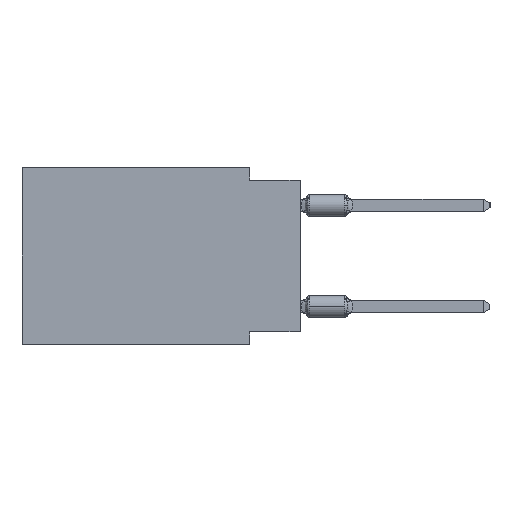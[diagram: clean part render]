
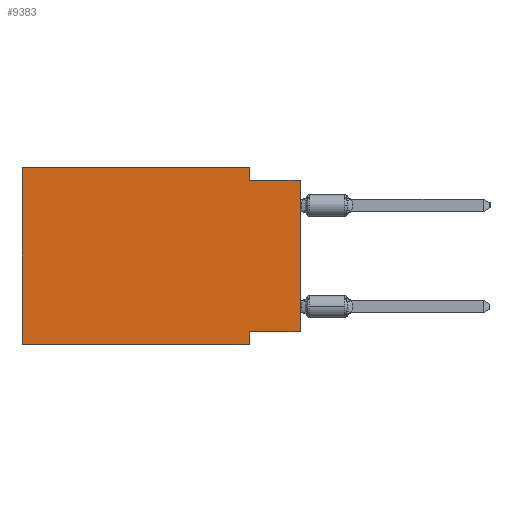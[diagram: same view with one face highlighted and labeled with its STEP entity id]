
A CAD part, left-side view. The second image highlights one B-rep face of the part: STEP entity #9383.
In plain terms, the highlighted planar face has unit normal (-1, 0, 0).
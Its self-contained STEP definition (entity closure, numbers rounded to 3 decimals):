
#22 = LINE ( 'NONE', #15636, #12544 ) ;
#81 = VERTEX_POINT ( 'NONE', #32226 ) ;
#788 = EDGE_LOOP ( 'NONE', ( #20646, #19501, #6830, #11508, #5586, #4826, #31515, #23797 ) ) ;
#2620 = EDGE_CURVE ( 'NONE', #30941, #81, #27450, .T. ) ;
#4728 = CARTESIAN_POINT ( 'NONE',  ( 0., 13.97, -8.89 ) ) ;
#4826 = ORIENTED_EDGE ( 'NONE', *, *, #15686, .T. ) ;
#4896 = CARTESIAN_POINT ( 'NONE',  ( 0., 0., -8.255 ) ) ;
#5426 = VECTOR ( 'NONE', #12375, 1000. ) ;
#5586 = ORIENTED_EDGE ( 'NONE', *, *, #15445, .F. ) ;
#5621 = LINE ( 'NONE', #7819, #14363 ) ;
#6531 = VECTOR ( 'NONE', #18871, 1000. ) ;
#6609 = LINE ( 'NONE', #20182, #5426 ) ;
#6830 = ORIENTED_EDGE ( 'NONE', *, *, #10685, .F. ) ;
#7659 = VECTOR ( 'NONE', #31366, 1000. ) ;
#7726 = LINE ( 'NONE', #18282, #7659 ) ;
#7819 = CARTESIAN_POINT ( 'NONE',  ( 0., 0., -0.635 ) ) ;
#7893 = VERTEX_POINT ( 'NONE', #19875 ) ;
#8503 = LINE ( 'NONE', #11541, #6531 ) ;
#9383 = ADVANCED_FACE ( 'NONE', ( #26511 ), #13760, .F. ) ;
#9607 = EDGE_CURVE ( 'NONE', #19633, #23455, #6609, .T. ) ;
#9655 = VERTEX_POINT ( 'NONE', #4896 ) ;
#10685 = EDGE_CURVE ( 'NONE', #23455, #26464, #8503, .T. ) ;
#10727 = CARTESIAN_POINT ( 'NONE',  ( 0., 13.97, 0. ) ) ;
#11388 = EDGE_CURVE ( 'NONE', #9655, #30941, #7726, .T. ) ;
#11508 = ORIENTED_EDGE ( 'NONE', *, *, #9607, .F. ) ;
#11541 = CARTESIAN_POINT ( 'NONE',  ( 0., 2.54, 0. ) ) ;
#11980 = CARTESIAN_POINT ( 'NONE',  ( 0., 2.54, -8.89 ) ) ;
#12375 = DIRECTION ( 'NONE',  ( 0., -1., 0. ) ) ;
#12544 = VECTOR ( 'NONE', #31264, 1000. ) ;
#13760 = PLANE ( 'NONE',  #29288 ) ;
#13778 = CARTESIAN_POINT ( 'NONE',  ( 0., 0., 0. ) ) ;
#13934 = DIRECTION ( 'NONE',  ( 1., 0., 0. ) ) ;
#14101 = CARTESIAN_POINT ( 'NONE',  ( 0., 13.97, 0. ) ) ;
#14363 = VECTOR ( 'NONE', #18198, 1000. ) ;
#14599 = CARTESIAN_POINT ( 'NONE',  ( 0., 2.54, -8.255 ) ) ;
#14922 = DIRECTION ( 'NONE',  ( 0., -1., 0. ) ) ;
#15088 = LINE ( 'NONE', #4728, #18521 ) ;
#15445 = EDGE_CURVE ( 'NONE', #19570, #19633, #22, .T. ) ;
#15636 = CARTESIAN_POINT ( 'NONE',  ( 0., 13.97, 0. ) ) ;
#15686 = EDGE_CURVE ( 'NONE', #19570, #81, #15088, .T. ) ;
#15997 = LINE ( 'NONE', #13778, #32471 ) ;
#17254 = DIRECTION ( 'NONE',  ( 0., 0., -1. ) ) ;
#18198 = DIRECTION ( 'NONE',  ( 0., -1., 0. ) ) ;
#18282 = CARTESIAN_POINT ( 'NONE',  ( 0., 0., -8.255 ) ) ;
#18521 = VECTOR ( 'NONE', #14922, 1000. ) ;
#18871 = DIRECTION ( 'NONE',  ( 0., 0., -1. ) ) ;
#19501 = ORIENTED_EDGE ( 'NONE', *, *, #33480, .F. ) ;
#19570 = VERTEX_POINT ( 'NONE', #25517 ) ;
#19633 = VERTEX_POINT ( 'NONE', #10727 ) ;
#19875 = CARTESIAN_POINT ( 'NONE',  ( 0., 0., -0.635 ) ) ;
#20182 = CARTESIAN_POINT ( 'NONE',  ( 0., 13.97, 0. ) ) ;
#20359 = VECTOR ( 'NONE', #17254, 1000. ) ;
#20646 = ORIENTED_EDGE ( 'NONE', *, *, #23192, .T. ) ;
#23192 = EDGE_CURVE ( 'NONE', #9655, #7893, #15997, .T. ) ;
#23455 = VERTEX_POINT ( 'NONE', #29573 ) ;
#23797 = ORIENTED_EDGE ( 'NONE', *, *, #11388, .F. ) ;
#24135 = DIRECTION ( 'NONE',  ( 0., 0., -1. ) ) ;
#25517 = CARTESIAN_POINT ( 'NONE',  ( 0., 13.97, -8.89 ) ) ;
#26176 = DIRECTION ( 'NONE',  ( 0., 0., 1. ) ) ;
#26464 = VERTEX_POINT ( 'NONE', #27019 ) ;
#26511 = FACE_OUTER_BOUND ( 'NONE', #788, .T. ) ;
#27019 = CARTESIAN_POINT ( 'NONE',  ( 0., 2.54, -0.635 ) ) ;
#27450 = LINE ( 'NONE', #11980, #20359 ) ;
#29288 = AXIS2_PLACEMENT_3D ( 'NONE', #14101, #13934, #24135 ) ;
#29573 = CARTESIAN_POINT ( 'NONE',  ( 0., 2.54, 0. ) ) ;
#30941 = VERTEX_POINT ( 'NONE', #14599 ) ;
#31264 = DIRECTION ( 'NONE',  ( 0., 0., 1. ) ) ;
#31366 = DIRECTION ( 'NONE',  ( 0., 1., 0. ) ) ;
#31515 = ORIENTED_EDGE ( 'NONE', *, *, #2620, .F. ) ;
#32226 = CARTESIAN_POINT ( 'NONE',  ( 0., 2.54, -8.89 ) ) ;
#32471 = VECTOR ( 'NONE', #26176, 1000. ) ;
#33480 = EDGE_CURVE ( 'NONE', #26464, #7893, #5621, .T. ) ;
